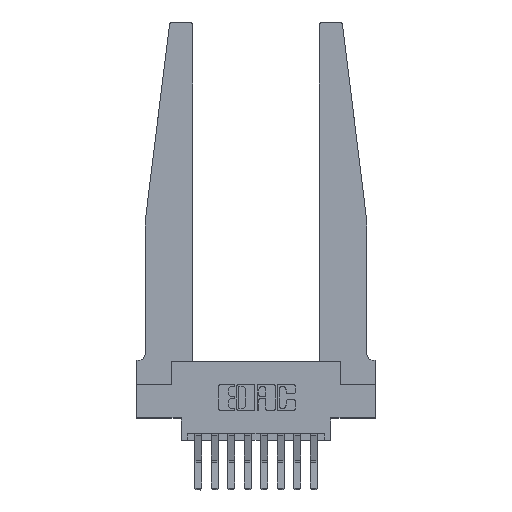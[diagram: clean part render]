
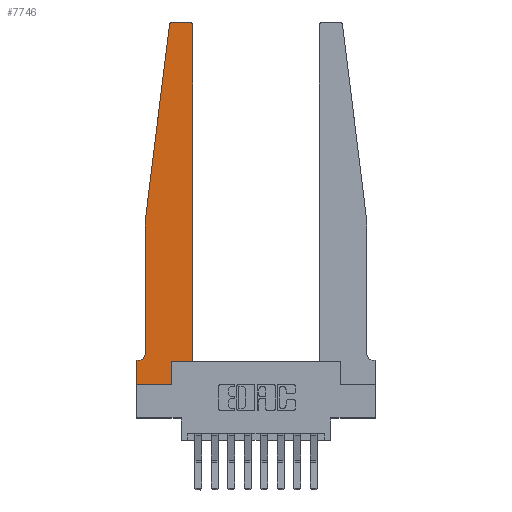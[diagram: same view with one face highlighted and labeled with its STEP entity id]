
A CAD part, top view. The second image highlights one B-rep face of the part: STEP entity #7746.
In plain terms, the highlighted planar face has unit normal (0, 0, 1).
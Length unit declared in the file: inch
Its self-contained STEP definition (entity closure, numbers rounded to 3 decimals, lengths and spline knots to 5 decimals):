
#39 = CARTESIAN_POINT ( 'NONE',  ( 0.425, 0.18, 0.37 ) ) ;
#375 = EDGE_CURVE ( 'NONE', #7976, #12443, #11286, .T. ) ;
#1053 = FACE_OUTER_BOUND ( 'NONE', #8513, .T. ) ;
#1256 = ORIENTED_EDGE ( 'NONE', *, *, #375, .T. ) ;
#1485 = ORIENTED_EDGE ( 'NONE', *, *, #1984, .T. ) ;
#1812 = VERTEX_POINT ( 'NONE', #6437 ) ;
#1957 = AXIS2_PLACEMENT_3D ( 'NONE', #9122, #2273, #10284 ) ;
#1984 = EDGE_CURVE ( 'NONE', #3177, #9672, #13781, .T. ) ;
#2002 = ORIENTED_EDGE ( 'NONE', *, *, #6603, .T. ) ;
#2273 = DIRECTION ( 'NONE',  ( 0., 0., 1. ) ) ;
#2279 = EDGE_CURVE ( 'NONE', #4429, #10230, #6787, .T. ) ;
#2509 = ORIENTED_EDGE ( 'NONE', *, *, #4831, .T. ) ;
#2641 = LINE ( 'NONE', #11852, #14473 ) ;
#2909 = DIRECTION ( 'NONE',  ( 0., 1., 0. ) ) ;
#2945 = ORIENTED_EDGE ( 'NONE', *, *, #5502, .T. ) ;
#2964 = CARTESIAN_POINT ( 'NONE',  ( 0., 0., 0.37 ) ) ;
#3177 = VERTEX_POINT ( 'NONE', #8937 ) ;
#3528 = ORIENTED_EDGE ( 'NONE', *, *, #4234, .T. ) ;
#3649 = PLANE ( 'NONE',  #4005 ) ;
#3919 = VECTOR ( 'NONE', #4553, 39.37008 ) ;
#4005 = AXIS2_PLACEMENT_3D ( 'NONE', #4742, #11668, #4785 ) ;
#4186 = LINE ( 'NONE', #5443, #6889 ) ;
#4234 = EDGE_CURVE ( 'NONE', #8547, #14379, #12105, .T. ) ;
#4239 = CARTESIAN_POINT ( 'NONE',  ( 0.015, 0.2375, 0.37 ) ) ;
#4429 = VERTEX_POINT ( 'NONE', #39 ) ;
#4553 = DIRECTION ( 'NONE',  ( 0., -1., 0. ) ) ;
#4601 = CARTESIAN_POINT ( 'NONE',  ( 0.065, 0.1875, 0.37 ) ) ;
#4742 = CARTESIAN_POINT ( 'NONE',  ( 0., 0.1875, 0.37 ) ) ;
#4770 = ORIENTED_EDGE ( 'NONE', *, *, #9371, .T. ) ;
#4785 = DIRECTION ( 'NONE',  ( 1., 0., 0. ) ) ;
#4831 = EDGE_CURVE ( 'NONE', #13475, #1812, #4186, .T. ) ;
#5188 = CARTESIAN_POINT ( 'NONE',  ( 0.2605, 0.18, 0.37 ) ) ;
#5406 = DIRECTION ( 'NONE',  ( -1., 0., 0. ) ) ;
#5443 = CARTESIAN_POINT ( 'NONE',  ( 0.065, 1.25, 0.37 ) ) ;
#5502 = EDGE_CURVE ( 'NONE', #12681, #13475, #8467, .T. ) ;
#5517 = ORIENTED_EDGE ( 'NONE', *, *, #8384, .T. ) ;
#5703 = CARTESIAN_POINT ( 'NONE',  ( 0.395, 2.72, 0.37 ) ) ;
#5971 = ORIENTED_EDGE ( 'NONE', *, *, #7410, .T. ) ;
#6181 = AXIS2_PLACEMENT_3D ( 'NONE', #4239, #12268, #5406 ) ;
#6402 = CIRCLE ( 'NONE', #11594, 0.03 ) ;
#6403 = CARTESIAN_POINT ( 'NONE',  ( 0.065, 0.2375, 0.37 ) ) ;
#6437 = CARTESIAN_POINT ( 'NONE',  ( 0.065, 1.25, 0.37 ) ) ;
#6531 = DIRECTION ( 'NONE',  ( -1., 0., 0. ) ) ;
#6603 = EDGE_CURVE ( 'NONE', #1812, #8547, #8961, .T. ) ;
#6678 = ORIENTED_EDGE ( 'NONE', *, *, #8780, .T. ) ;
#6787 = LINE ( 'NONE', #14321, #9457 ) ;
#6837 = DIRECTION ( 'NONE',  ( 1., 0., 0. ) ) ;
#6889 = VECTOR ( 'NONE', #14613, 39.37008 ) ;
#7410 = EDGE_CURVE ( 'NONE', #8422, #12681, #11083, .T. ) ;
#7746 = ADVANCED_FACE ( 'NONE', ( #1053 ), #3649, .T. ) ;
#7878 = VECTOR ( 'NONE', #9936, 39.37008 ) ;
#7976 = VERTEX_POINT ( 'NONE', #8648 ) ;
#7979 = VECTOR ( 'NONE', #13780, 39.37008 ) ;
#8037 = VECTOR ( 'NONE', #6531, 39.37008 ) ;
#8375 = CARTESIAN_POINT ( 'NONE',  ( 0.425, 2.72, 0.37 ) ) ;
#8384 = EDGE_CURVE ( 'NONE', #9672, #7976, #2641, .T. ) ;
#8422 = VERTEX_POINT ( 'NONE', #14212 ) ;
#8466 = ORIENTED_EDGE ( 'NONE', *, *, #2279, .T. ) ;
#8467 = CIRCLE ( 'NONE', #1957, 0.03 ) ;
#8513 = EDGE_LOOP ( 'NONE', ( #5971, #2945, #2509, #2002, #3528, #4770, #1485, #5517, #1256, #9586, #8466, #6678 ) ) ;
#8547 = VERTEX_POINT ( 'NONE', #6403 ) ;
#8593 = VECTOR ( 'NONE', #13453, 39.37008 ) ;
#8648 = CARTESIAN_POINT ( 'NONE',  ( 0.2605, 0., 0.37 ) ) ;
#8780 = EDGE_CURVE ( 'NONE', #10230, #8422, #6402, .T. ) ;
#8937 = CARTESIAN_POINT ( 'NONE',  ( 0., 0.1875, 0.37 ) ) ;
#8961 = LINE ( 'NONE', #12305, #8593 ) ;
#9122 = CARTESIAN_POINT ( 'NONE',  ( 0.27653, 2.72, 0.37 ) ) ;
#9371 = EDGE_CURVE ( 'NONE', #14379, #3177, #14091, .T. ) ;
#9457 = VECTOR ( 'NONE', #2909, 39.37008 ) ;
#9586 = ORIENTED_EDGE ( 'NONE', *, *, #13393, .T. ) ;
#9672 = VERTEX_POINT ( 'NONE', #2964 ) ;
#9689 = CARTESIAN_POINT ( 'NONE',  ( 0.425, 0.18, 0.37 ) ) ;
#9739 = DIRECTION ( 'NONE',  ( 1., 0., 0. ) ) ;
#9936 = DIRECTION ( 'NONE',  ( 0., 1., 0. ) ) ;
#10230 = VERTEX_POINT ( 'NONE', #8375 ) ;
#10284 = DIRECTION ( 'NONE',  ( 1., 0., 0. ) ) ;
#10560 = CARTESIAN_POINT ( 'NONE',  ( 0.015, 0.1875, 0.37 ) ) ;
#11072 = CARTESIAN_POINT ( 'NONE',  ( 0.25, 2.75, 0.37 ) ) ;
#11083 = LINE ( 'NONE', #11072, #8037 ) ;
#11286 = LINE ( 'NONE', #5188, #7878 ) ;
#11303 = LINE ( 'NONE', #9689, #14006 ) ;
#11594 = AXIS2_PLACEMENT_3D ( 'NONE', #5703, #13707, #6837 ) ;
#11668 = DIRECTION ( 'NONE',  ( 0., 0., 1. ) ) ;
#11852 = CARTESIAN_POINT ( 'NONE',  ( 0., 0., 0.37 ) ) ;
#12105 = CIRCLE ( 'NONE', #6181, 0.05 ) ;
#12268 = DIRECTION ( 'NONE',  ( 0., 0., -1. ) ) ;
#12305 = CARTESIAN_POINT ( 'NONE',  ( 0.065, 1.25, 0.37 ) ) ;
#12443 = VERTEX_POINT ( 'NONE', #12827 ) ;
#12681 = VERTEX_POINT ( 'NONE', #12812 ) ;
#12812 = CARTESIAN_POINT ( 'NONE',  ( 0.27653, 2.75, 0.37 ) ) ;
#12827 = CARTESIAN_POINT ( 'NONE',  ( 0.2605, 0.18, 0.37 ) ) ;
#12947 = DIRECTION ( 'NONE',  ( 1., 0., 0. ) ) ;
#13393 = EDGE_CURVE ( 'NONE', #12443, #4429, #11303, .T. ) ;
#13453 = DIRECTION ( 'NONE',  ( 0., -1., 0. ) ) ;
#13475 = VERTEX_POINT ( 'NONE', #14457 ) ;
#13685 = CARTESIAN_POINT ( 'NONE',  ( 0., 0., 0.37 ) ) ;
#13707 = DIRECTION ( 'NONE',  ( 0., 0., 1. ) ) ;
#13780 = DIRECTION ( 'NONE',  ( -1., 0., 0. ) ) ;
#13781 = LINE ( 'NONE', #13685, #3919 ) ;
#14006 = VECTOR ( 'NONE', #9739, 39.37008 ) ;
#14091 = LINE ( 'NONE', #4601, #7979 ) ;
#14212 = CARTESIAN_POINT ( 'NONE',  ( 0.395, 2.75, 0.37 ) ) ;
#14321 = CARTESIAN_POINT ( 'NONE',  ( 0.425, 0.18, 0.37 ) ) ;
#14379 = VERTEX_POINT ( 'NONE', #10560 ) ;
#14457 = CARTESIAN_POINT ( 'NONE',  ( 0.24675, 2.72367, 0.37 ) ) ;
#14473 = VECTOR ( 'NONE', #12947, 39.37008 ) ;
#14613 = DIRECTION ( 'NONE',  ( -0.122, -0.992, 0. ) ) ;
